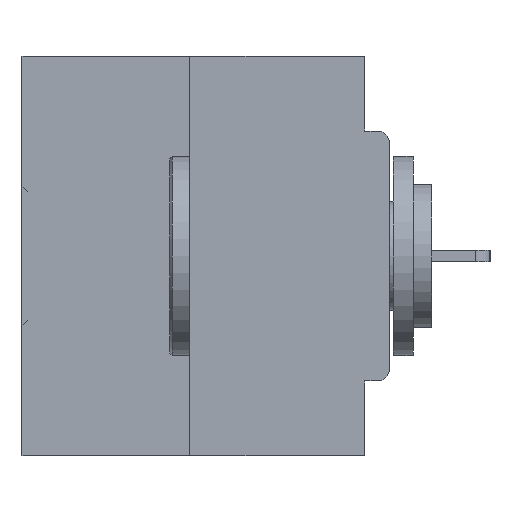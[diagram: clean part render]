
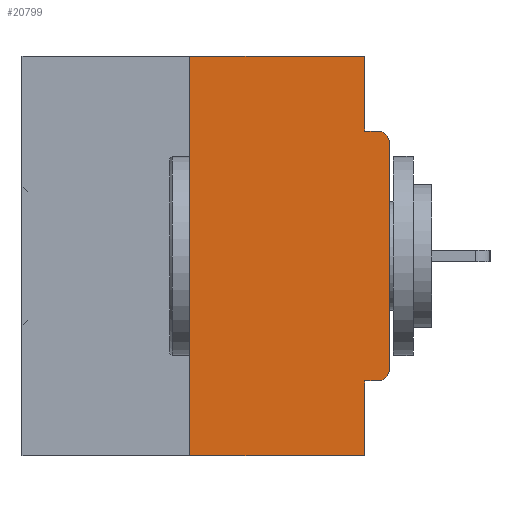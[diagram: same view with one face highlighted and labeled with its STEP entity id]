
A CAD part, left-side view. The second image highlights one B-rep face of the part: STEP entity #20799.
In plain terms, the highlighted planar face has unit normal (-1, 0, 0).
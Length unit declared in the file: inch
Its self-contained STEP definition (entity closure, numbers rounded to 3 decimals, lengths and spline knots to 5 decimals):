
#86 = VECTOR ( 'NONE', #7186, 39.37008 ) ;
#268 = VERTEX_POINT ( 'NONE', #2227 ) ;
#2227 = CARTESIAN_POINT ( 'NONE',  ( 0., 0.031, -0.5 ) ) ;
#2381 = VERTEX_POINT ( 'NONE', #25147 ) ;
#2950 = VERTEX_POINT ( 'NONE', #12530 ) ;
#3160 = FACE_OUTER_BOUND ( 'NONE', #14689, .T. ) ;
#3469 = ORIENTED_EDGE ( 'NONE', *, *, #37585, .T. ) ;
#3989 = AXIS2_PLACEMENT_3D ( 'NONE', #6209, #30805, #37501 ) ;
#4305 = VECTOR ( 'NONE', #31690, 39.37008 ) ;
#4624 = ORIENTED_EDGE ( 'NONE', *, *, #24257, .F. ) ;
#4867 = LINE ( 'NONE', #35753, #11331 ) ;
#5274 = EDGE_CURVE ( 'NONE', #27357, #8602, #10658, .T. ) ;
#5649 = CIRCLE ( 'NONE', #20074, 0.015 ) ;
#6158 = CARTESIAN_POINT ( 'NONE',  ( 0., 0.031, -0.0935 ) ) ;
#6209 = CARTESIAN_POINT ( 'NONE',  ( 0., 0.46, 0. ) ) ;
#6468 = CARTESIAN_POINT ( 'NONE',  ( 0., 0., -0.1085 ) ) ;
#6533 = VECTOR ( 'NONE', #9569, 39.37008 ) ;
#6827 = VECTOR ( 'NONE', #22797, 39.37008 ) ;
#6899 = LINE ( 'NONE', #19335, #4305 ) ;
#7186 = DIRECTION ( 'NONE',  ( 0., 0., 1. ) ) ;
#7298 = DIRECTION ( 'NONE',  ( 0., -1., 0. ) ) ;
#7309 = EDGE_CURVE ( 'NONE', #27357, #268, #26009, .T. ) ;
#7314 = EDGE_CURVE ( 'NONE', #2381, #2950, #6899, .T. ) ;
#7479 = CIRCLE ( 'NONE', #21809, 0.015 ) ;
#8602 = VERTEX_POINT ( 'NONE', #15042 ) ;
#8914 = LINE ( 'NONE', #27806, #18062 ) ;
#9494 = VERTEX_POINT ( 'NONE', #37494 ) ;
#9569 = DIRECTION ( 'NONE',  ( 0., -1., 0. ) ) ;
#9683 = CARTESIAN_POINT ( 'NONE',  ( 0., 0.031, 0. ) ) ;
#10658 = LINE ( 'NONE', #19630, #86 ) ;
#10855 = CARTESIAN_POINT ( 'NONE',  ( 0., 0.015, -0.1085 ) ) ;
#11175 = VECTOR ( 'NONE', #37300, 39.37008 ) ;
#11331 = VECTOR ( 'NONE', #39247, 39.37008 ) ;
#11507 = VECTOR ( 'NONE', #7298, 39.37008 ) ;
#11940 = VERTEX_POINT ( 'NONE', #6468 ) ;
#12530 = CARTESIAN_POINT ( 'NONE',  ( 0., 0.031, -0.4065 ) ) ;
#12955 = CARTESIAN_POINT ( 'NONE',  ( 0., 0.015, -0.0935 ) ) ;
#14689 = EDGE_LOOP ( 'NONE', ( #4624, #36417, #22931, #35897, #31188, #28443, #3469, #28244, #15850, #24494 ) ) ;
#15042 = CARTESIAN_POINT ( 'NONE',  ( 0., 0.25, 0. ) ) ;
#15850 = ORIENTED_EDGE ( 'NONE', *, *, #17581, .F. ) ;
#17581 = EDGE_CURVE ( 'NONE', #21280, #25405, #31305, .T. ) ;
#18062 = VECTOR ( 'NONE', #18094, 39.37008 ) ;
#18094 = DIRECTION ( 'NONE',  ( 0., 0., 1. ) ) ;
#18346 = CARTESIAN_POINT ( 'NONE',  ( 0., 0., -0.0935 ) ) ;
#18453 = PLANE ( 'NONE',  #3989 ) ;
#19335 = CARTESIAN_POINT ( 'NONE',  ( 0., 0., -0.4065 ) ) ;
#19411 = DIRECTION ( 'NONE',  ( -1., 0., 0. ) ) ;
#19630 = CARTESIAN_POINT ( 'NONE',  ( 0., 0.25, 0. ) ) ;
#19754 = LINE ( 'NONE', #26228, #6827 ) ;
#20074 = AXIS2_PLACEMENT_3D ( 'NONE', #10855, #19411, #28527 ) ;
#20618 = CARTESIAN_POINT ( 'NONE',  ( 0., 0.25, -0.5 ) ) ;
#20757 = CARTESIAN_POINT ( 'NONE',  ( 0., 0.015, -0.3915 ) ) ;
#20779 = EDGE_CURVE ( 'NONE', #9494, #21280, #40165, .T. ) ;
#20799 = ADVANCED_FACE ( 'NONE', ( #3160 ), #18453, .F. ) ;
#21280 = VERTEX_POINT ( 'NONE', #6158 ) ;
#21809 = AXIS2_PLACEMENT_3D ( 'NONE', #20757, #33111, #39427 ) ;
#22797 = DIRECTION ( 'NONE',  ( 0., -1., 0. ) ) ;
#22931 = ORIENTED_EDGE ( 'NONE', *, *, #7309, .T. ) ;
#24257 = EDGE_CURVE ( 'NONE', #8602, #9494, #19754, .T. ) ;
#24491 = EDGE_CURVE ( 'NONE', #2381, #25742, #7479, .T. ) ;
#24494 = ORIENTED_EDGE ( 'NONE', *, *, #20779, .F. ) ;
#25147 = CARTESIAN_POINT ( 'NONE',  ( 0., 0.015, -0.4065 ) ) ;
#25405 = VERTEX_POINT ( 'NONE', #12955 ) ;
#25742 = VERTEX_POINT ( 'NONE', #33221 ) ;
#26009 = LINE ( 'NONE', #29446, #11507 ) ;
#26228 = CARTESIAN_POINT ( 'NONE',  ( 0., 0.46, 0. ) ) ;
#27357 = VERTEX_POINT ( 'NONE', #20618 ) ;
#27806 = CARTESIAN_POINT ( 'NONE',  ( 0., 0., 0. ) ) ;
#28244 = ORIENTED_EDGE ( 'NONE', *, *, #30651, .T. ) ;
#28443 = ORIENTED_EDGE ( 'NONE', *, *, #24491, .T. ) ;
#28527 = DIRECTION ( 'NONE',  ( 0., 0., -1. ) ) ;
#29446 = CARTESIAN_POINT ( 'NONE',  ( 0., 0.46, -0.5 ) ) ;
#30651 = EDGE_CURVE ( 'NONE', #11940, #25405, #5649, .T. ) ;
#30805 = DIRECTION ( 'NONE',  ( 1., 0., 0. ) ) ;
#31188 = ORIENTED_EDGE ( 'NONE', *, *, #7314, .F. ) ;
#31305 = LINE ( 'NONE', #18346, #6533 ) ;
#31690 = DIRECTION ( 'NONE',  ( 0., 1., 0. ) ) ;
#32495 = EDGE_CURVE ( 'NONE', #2950, #268, #4867, .T. ) ;
#33111 = DIRECTION ( 'NONE',  ( -1., 0., 0. ) ) ;
#33221 = CARTESIAN_POINT ( 'NONE',  ( 0., 0., -0.3915 ) ) ;
#35753 = CARTESIAN_POINT ( 'NONE',  ( 0., 0.031, -0.5 ) ) ;
#35897 = ORIENTED_EDGE ( 'NONE', *, *, #32495, .F. ) ;
#36417 = ORIENTED_EDGE ( 'NONE', *, *, #5274, .F. ) ;
#37300 = DIRECTION ( 'NONE',  ( 0., 0., -1. ) ) ;
#37494 = CARTESIAN_POINT ( 'NONE',  ( 0., 0.031, 0. ) ) ;
#37501 = DIRECTION ( 'NONE',  ( 0., 0., -1. ) ) ;
#37585 = EDGE_CURVE ( 'NONE', #25742, #11940, #8914, .T. ) ;
#39247 = DIRECTION ( 'NONE',  ( 0., 0., -1. ) ) ;
#39427 = DIRECTION ( 'NONE',  ( 0., 0., -1. ) ) ;
#40165 = LINE ( 'NONE', #9683, #11175 ) ;
